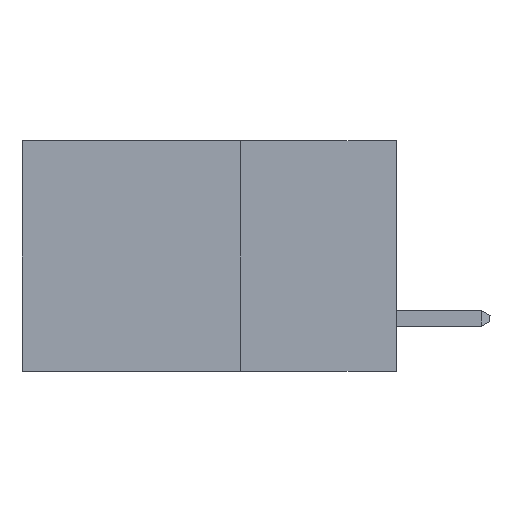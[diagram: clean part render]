
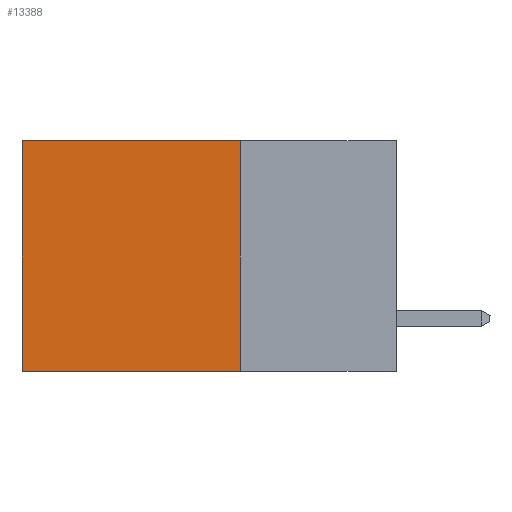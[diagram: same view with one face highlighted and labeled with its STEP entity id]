
A CAD part, left-side view. The second image highlights one B-rep face of the part: STEP entity #13388.
In plain terms, the highlighted planar face has unit normal (-1, 0, 0).
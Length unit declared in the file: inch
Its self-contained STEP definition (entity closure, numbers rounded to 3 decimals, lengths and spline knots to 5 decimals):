
#1157 = ORIENTED_EDGE ( 'NONE', *, *, #11040, .F. ) ;
#1621 = CARTESIAN_POINT ( 'NONE',  ( 0.2615, 0.25, 0. ) ) ;
#2213 = CARTESIAN_POINT ( 'NONE',  ( 0.2615, 0.25, -0.37 ) ) ;
#2508 = CARTESIAN_POINT ( 'NONE',  ( 0.2615, 0.25, -0.37 ) ) ;
#2932 = DIRECTION ( 'NONE',  ( 0., 1., 0. ) ) ;
#3061 = CARTESIAN_POINT ( 'NONE',  ( 0.2615, 0.25, 0. ) ) ;
#4284 = LINE ( 'NONE', #5361, #15119 ) ;
#4424 = VERTEX_POINT ( 'NONE', #11466 ) ;
#5361 = CARTESIAN_POINT ( 'NONE',  ( 0.2615, 0.25, -0.37 ) ) ;
#5539 = EDGE_CURVE ( 'NONE', #6460, #8569, #9682, .T. ) ;
#5894 = VECTOR ( 'NONE', #2932, 39.37008 ) ;
#6068 = DIRECTION ( 'NONE',  ( 0., 0., -1. ) ) ;
#6442 = DIRECTION ( 'NONE',  ( 1., 0., 0. ) ) ;
#6460 = VERTEX_POINT ( 'NONE', #1621 ) ;
#6620 = EDGE_CURVE ( 'NONE', #14536, #4424, #9414, .T. ) ;
#7790 = ORIENTED_EDGE ( 'NONE', *, *, #5539, .T. ) ;
#7990 = ORIENTED_EDGE ( 'NONE', *, *, #6620, .F. ) ;
#8569 = VERTEX_POINT ( 'NONE', #16682 ) ;
#9414 = LINE ( 'NONE', #2508, #16884 ) ;
#9682 = LINE ( 'NONE', #3061, #5894 ) ;
#11040 = EDGE_CURVE ( 'NONE', #6460, #14536, #4284, .T. ) ;
#11466 = CARTESIAN_POINT ( 'NONE',  ( 0.2615, 0.6, -0.37 ) ) ;
#11567 = LINE ( 'NONE', #15977, #14845 ) ;
#11805 = CARTESIAN_POINT ( 'NONE',  ( 0.2615, 0.25, -0.37 ) ) ;
#12199 = FACE_OUTER_BOUND ( 'NONE', #13826, .T. ) ;
#13215 = EDGE_CURVE ( 'NONE', #8569, #4424, #11567, .T. ) ;
#13388 = ADVANCED_FACE ( 'NONE', ( #12199 ), #17573, .F. ) ;
#13826 = EDGE_LOOP ( 'NONE', ( #14817, #7990, #1157, #7790 ) ) ;
#14536 = VERTEX_POINT ( 'NONE', #11805 ) ;
#14817 = ORIENTED_EDGE ( 'NONE', *, *, #13215, .T. ) ;
#14845 = VECTOR ( 'NONE', #6068, 39.37008 ) ;
#15119 = VECTOR ( 'NONE', #15265, 39.37008 ) ;
#15144 = DIRECTION ( 'NONE',  ( 0., 1., 0. ) ) ;
#15265 = DIRECTION ( 'NONE',  ( 0., 0., -1. ) ) ;
#15814 = AXIS2_PLACEMENT_3D ( 'NONE', #2213, #6442, #16339 ) ;
#15977 = CARTESIAN_POINT ( 'NONE',  ( 0.2615, 0.6, -0.37 ) ) ;
#16339 = DIRECTION ( 'NONE',  ( 0., 0., -1. ) ) ;
#16682 = CARTESIAN_POINT ( 'NONE',  ( 0.2615, 0.6, 0. ) ) ;
#16884 = VECTOR ( 'NONE', #15144, 39.37008 ) ;
#17573 = PLANE ( 'NONE',  #15814 ) ;
